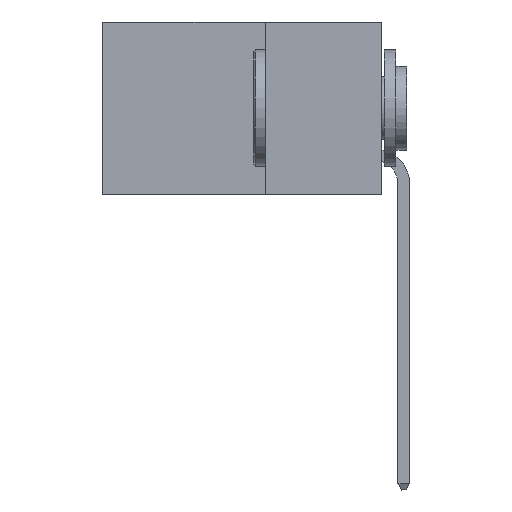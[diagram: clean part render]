
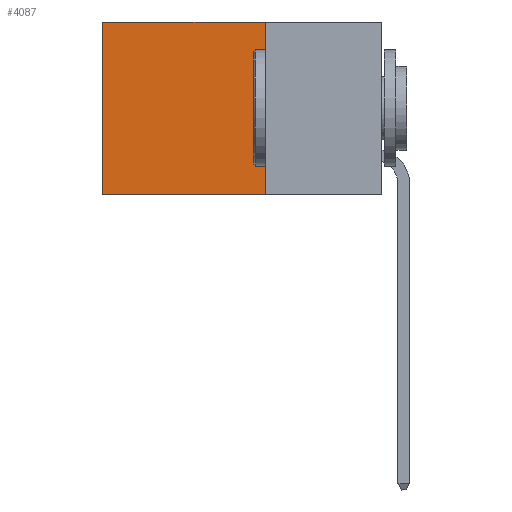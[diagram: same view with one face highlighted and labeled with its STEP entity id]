
A CAD part, left-side view. The second image highlights one B-rep face of the part: STEP entity #4087.
In plain terms, the highlighted planar face has unit normal (-1, 0, 0).
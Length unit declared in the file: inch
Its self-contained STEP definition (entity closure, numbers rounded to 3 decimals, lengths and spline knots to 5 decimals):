
#1397 = VERTEX_POINT ( 'NONE', #40743 ) ;
#2952 = CARTESIAN_POINT ( 'NONE',  ( 0.2875, 0.6, 0. ) ) ;
#3625 = DIRECTION ( 'NONE',  ( 0., 0., -1. ) ) ;
#4087 = ADVANCED_FACE ( 'NONE', ( #30399 ), #24875, .F. ) ;
#4769 = DIRECTION ( 'NONE',  ( 0., 0., -1. ) ) ;
#9599 = DIRECTION ( 'NONE',  ( 0., 0., -1. ) ) ;
#9851 = CARTESIAN_POINT ( 'NONE',  ( 0.2875, 0.25, -0.37 ) ) ;
#10458 = VERTEX_POINT ( 'NONE', #30646 ) ;
#10577 = EDGE_CURVE ( 'NONE', #22542, #10458, #30689, .T. ) ;
#12065 = EDGE_CURVE ( 'NONE', #29783, #10458, #21759, .T. ) ;
#12087 = VECTOR ( 'NONE', #9599, 39.37008 ) ;
#12862 = DIRECTION ( 'NONE',  ( 0., 1., 0. ) ) ;
#14366 = VECTOR ( 'NONE', #37999, 39.37008 ) ;
#15574 = CARTESIAN_POINT ( 'NONE',  ( 0.2875, 0.25, 0. ) ) ;
#16147 = ORIENTED_EDGE ( 'NONE', *, *, #10577, .F. ) ;
#17064 = ORIENTED_EDGE ( 'NONE', *, *, #12065, .T. ) ;
#18933 = EDGE_CURVE ( 'NONE', #1397, #29783, #33511, .T. ) ;
#21054 = EDGE_LOOP ( 'NONE', ( #17064, #16147, #37556, #24931 ) ) ;
#21138 = CARTESIAN_POINT ( 'NONE',  ( 0.2875, 0.25, 0. ) ) ;
#21759 = LINE ( 'NONE', #2952, #12087 ) ;
#22542 = VERTEX_POINT ( 'NONE', #37671 ) ;
#22967 = CARTESIAN_POINT ( 'NONE',  ( 0.2875, 0.6, 0. ) ) ;
#23813 = VECTOR ( 'NONE', #12862, 39.37008 ) ;
#24875 = PLANE ( 'NONE',  #36613 ) ;
#24931 = ORIENTED_EDGE ( 'NONE', *, *, #18933, .T. ) ;
#27384 = LINE ( 'NONE', #32889, #27934 ) ;
#27934 = VECTOR ( 'NONE', #3625, 39.37008 ) ;
#29783 = VERTEX_POINT ( 'NONE', #22967 ) ;
#30399 = FACE_OUTER_BOUND ( 'NONE', #21054, .T. ) ;
#30646 = CARTESIAN_POINT ( 'NONE',  ( 0.2875, 0.6, -0.37 ) ) ;
#30689 = LINE ( 'NONE', #9851, #14366 ) ;
#32889 = CARTESIAN_POINT ( 'NONE',  ( 0.2875, 0.25, 0. ) ) ;
#33511 = LINE ( 'NONE', #15574, #23813 ) ;
#36613 = AXIS2_PLACEMENT_3D ( 'NONE', #21138, #40850, #4769 ) ;
#37556 = ORIENTED_EDGE ( 'NONE', *, *, #37927, .F. ) ;
#37671 = CARTESIAN_POINT ( 'NONE',  ( 0.2875, 0.25, -0.37 ) ) ;
#37927 = EDGE_CURVE ( 'NONE', #1397, #22542, #27384, .T. ) ;
#37999 = DIRECTION ( 'NONE',  ( 0., 1., 0. ) ) ;
#40743 = CARTESIAN_POINT ( 'NONE',  ( 0.2875, 0.25, 0. ) ) ;
#40850 = DIRECTION ( 'NONE',  ( 1., 0., 0. ) ) ;
